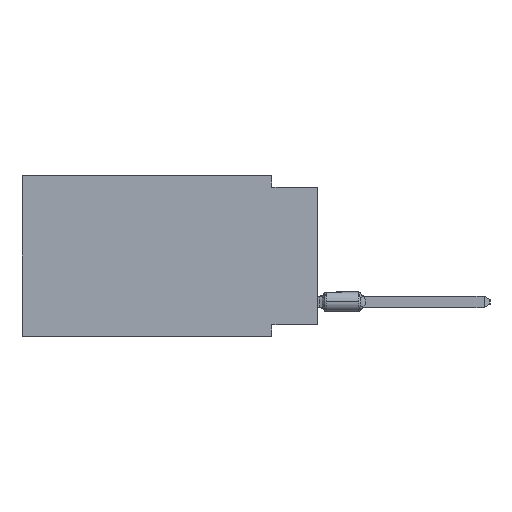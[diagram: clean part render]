
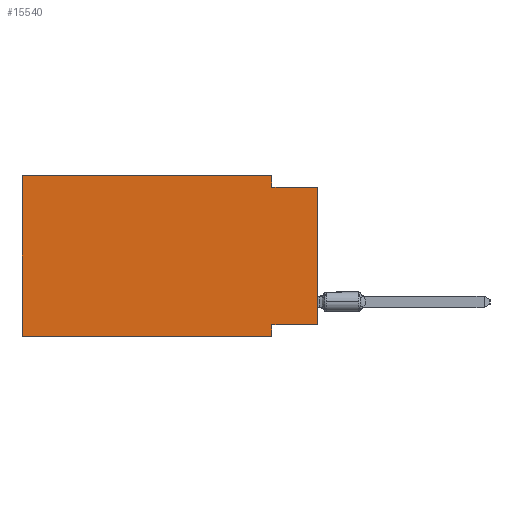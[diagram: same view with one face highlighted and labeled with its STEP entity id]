
A CAD part, left-side view. The second image highlights one B-rep face of the part: STEP entity #15540.
In plain terms, the highlighted planar face has unit normal (-1, 0, 0).
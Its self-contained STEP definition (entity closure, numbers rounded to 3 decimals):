
#363 = CARTESIAN_POINT ( 'NONE',  ( 0., 0., -8.255 ) ) ;
#462 = LINE ( 'NONE', #11254, #17085 ) ;
#1415 = VERTEX_POINT ( 'NONE', #20950 ) ;
#1462 = EDGE_CURVE ( 'NONE', #16064, #27051, #4047, .T. ) ;
#2163 = LINE ( 'NONE', #18787, #5033 ) ;
#3068 = DIRECTION ( 'NONE',  ( 0., 0., -1. ) ) ;
#3083 = DIRECTION ( 'NONE',  ( 0., 0., 1. ) ) ;
#4047 = LINE ( 'NONE', #10416, #7303 ) ;
#4651 = CARTESIAN_POINT ( 'NONE',  ( 0., 2.54, -0.635 ) ) ;
#5033 = VECTOR ( 'NONE', #6178, 1000. ) ;
#5298 = DIRECTION ( 'NONE',  ( 0., -1., 0. ) ) ;
#5414 = PLANE ( 'NONE',  #10363 ) ;
#5534 = ORIENTED_EDGE ( 'NONE', *, *, #26977, .F. ) ;
#6178 = DIRECTION ( 'NONE',  ( 0., 0., -1. ) ) ;
#6211 = EDGE_CURVE ( 'NONE', #16064, #11161, #462, .T. ) ;
#6859 = EDGE_CURVE ( 'NONE', #1415, #20795, #25711, .T. ) ;
#7011 = VERTEX_POINT ( 'NONE', #26244 ) ;
#7087 = LINE ( 'NONE', #19851, #7703 ) ;
#7303 = VECTOR ( 'NONE', #8344, 1000. ) ;
#7378 = CARTESIAN_POINT ( 'NONE',  ( 0., 2.54, -8.89 ) ) ;
#7703 = VECTOR ( 'NONE', #26327, 1000. ) ;
#7734 = VERTEX_POINT ( 'NONE', #4651 ) ;
#8344 = DIRECTION ( 'NONE',  ( 0., -1., 0. ) ) ;
#8361 = EDGE_CURVE ( 'NONE', #11161, #25738, #22201, .T. ) ;
#10154 = ORIENTED_EDGE ( 'NONE', *, *, #6211, .F. ) ;
#10363 = AXIS2_PLACEMENT_3D ( 'NONE', #24678, #24531, #3068 ) ;
#10416 = CARTESIAN_POINT ( 'NONE',  ( 0., 16.383, -8.89 ) ) ;
#10512 = CARTESIAN_POINT ( 'NONE',  ( 0., 16.383, -8.89 ) ) ;
#11161 = VERTEX_POINT ( 'NONE', #16361 ) ;
#11254 = CARTESIAN_POINT ( 'NONE',  ( 0., 16.383, 0. ) ) ;
#11587 = ORIENTED_EDGE ( 'NONE', *, *, #19572, .T. ) ;
#13449 = EDGE_LOOP ( 'NONE', ( #11587, #5534, #16208, #16345, #10154, #24380, #19835, #19202 ) ) ;
#14187 = EDGE_CURVE ( 'NONE', #20795, #27051, #17911, .T. ) ;
#14681 = LINE ( 'NONE', #23676, #16984 ) ;
#15036 = EDGE_CURVE ( 'NONE', #25738, #7734, #2163, .T. ) ;
#15089 = CARTESIAN_POINT ( 'NONE',  ( 0., 2.54, -8.89 ) ) ;
#15540 = ADVANCED_FACE ( 'NONE', ( #22183 ), #5414, .F. ) ;
#16064 = VERTEX_POINT ( 'NONE', #10512 ) ;
#16208 = ORIENTED_EDGE ( 'NONE', *, *, #15036, .F. ) ;
#16345 = ORIENTED_EDGE ( 'NONE', *, *, #8361, .F. ) ;
#16361 = CARTESIAN_POINT ( 'NONE',  ( 0., 16.383, 0. ) ) ;
#16984 = VECTOR ( 'NONE', #23544, 1000. ) ;
#17085 = VECTOR ( 'NONE', #3083, 1000. ) ;
#17911 = LINE ( 'NONE', #7378, #25767 ) ;
#18787 = CARTESIAN_POINT ( 'NONE',  ( 0., 2.54, 0. ) ) ;
#18935 = VECTOR ( 'NONE', #21573, 1000. ) ;
#19202 = ORIENTED_EDGE ( 'NONE', *, *, #6859, .F. ) ;
#19453 = VECTOR ( 'NONE', #5298, 1000. ) ;
#19572 = EDGE_CURVE ( 'NONE', #1415, #7011, #7087, .T. ) ;
#19835 = ORIENTED_EDGE ( 'NONE', *, *, #14187, .F. ) ;
#19851 = CARTESIAN_POINT ( 'NONE',  ( 0., 0., 0. ) ) ;
#20795 = VERTEX_POINT ( 'NONE', #22192 ) ;
#20950 = CARTESIAN_POINT ( 'NONE',  ( 0., 0., -8.255 ) ) ;
#21573 = DIRECTION ( 'NONE',  ( 0., 1., 0. ) ) ;
#22183 = FACE_OUTER_BOUND ( 'NONE', #13449, .T. ) ;
#22192 = CARTESIAN_POINT ( 'NONE',  ( 0., 2.54, -8.255 ) ) ;
#22201 = LINE ( 'NONE', #22764, #19453 ) ;
#22764 = CARTESIAN_POINT ( 'NONE',  ( 0., 16.383, 0. ) ) ;
#23544 = DIRECTION ( 'NONE',  ( 0., -1., 0. ) ) ;
#23676 = CARTESIAN_POINT ( 'NONE',  ( 0., 0., -0.635 ) ) ;
#24285 = DIRECTION ( 'NONE',  ( 0., 0., -1. ) ) ;
#24380 = ORIENTED_EDGE ( 'NONE', *, *, #1462, .T. ) ;
#24531 = DIRECTION ( 'NONE',  ( 1., 0., 0. ) ) ;
#24678 = CARTESIAN_POINT ( 'NONE',  ( 0., 16.383, 0. ) ) ;
#25711 = LINE ( 'NONE', #363, #18935 ) ;
#25738 = VERTEX_POINT ( 'NONE', #26753 ) ;
#25767 = VECTOR ( 'NONE', #24285, 1000. ) ;
#26244 = CARTESIAN_POINT ( 'NONE',  ( 0., 0., -0.635 ) ) ;
#26327 = DIRECTION ( 'NONE',  ( 0., 0., 1. ) ) ;
#26753 = CARTESIAN_POINT ( 'NONE',  ( 0., 2.54, 0. ) ) ;
#26977 = EDGE_CURVE ( 'NONE', #7734, #7011, #14681, .T. ) ;
#27051 = VERTEX_POINT ( 'NONE', #15089 ) ;
